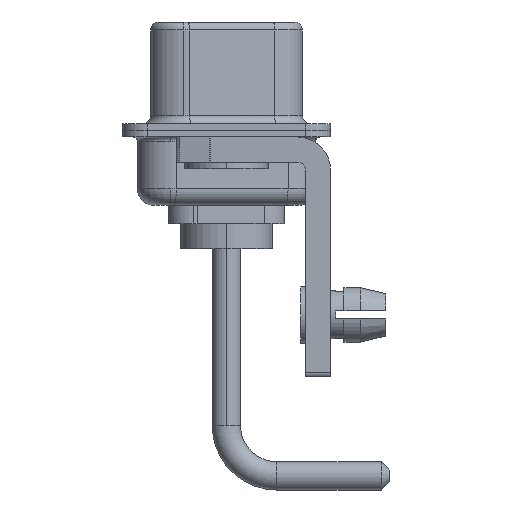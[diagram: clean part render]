
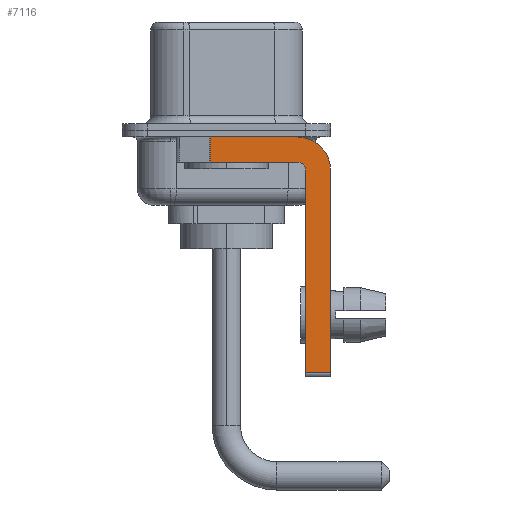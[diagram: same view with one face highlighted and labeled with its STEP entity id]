
A CAD part, left-side view. The second image highlights one B-rep face of the part: STEP entity #7116.
In plain terms, the highlighted planar face has unit normal (-1, 0, 0).
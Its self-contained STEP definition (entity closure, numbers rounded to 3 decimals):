
#137 = CARTESIAN_POINT ( 'NONE',  ( -2.9, -4.75, -14.55 ) ) ;
#662 = AXIS2_PLACEMENT_3D ( 'NONE', #3367, #9069, #10191 ) ;
#943 = CIRCLE ( 'NONE', #3325, 0.5 ) ;
#1096 = CARTESIAN_POINT ( 'NONE',  ( -2.9, -6.25, -2.4 ) ) ;
#1313 = CARTESIAN_POINT ( 'NONE',  ( -2.9, -4.75, -2.4 ) ) ;
#1391 = DIRECTION ( 'NONE',  ( 0., -1., 0. ) ) ;
#1583 = VERTEX_POINT ( 'NONE', #15794 ) ;
#1689 = EDGE_CURVE ( 'NONE', #6474, #12351, #4305, .T. ) ;
#1691 = VERTEX_POINT ( 'NONE', #13336 ) ;
#1703 = CARTESIAN_POINT ( 'NONE',  ( -2.9, -4.25, -2.4 ) ) ;
#1870 = FACE_OUTER_BOUND ( 'NONE', #11598, .T. ) ;
#2334 = EDGE_CURVE ( 'NONE', #17077, #16616, #3514, .T. ) ;
#2384 = ORIENTED_EDGE ( 'NONE', *, *, #13495, .F. ) ;
#2458 = LINE ( 'NONE', #12449, #12883 ) ;
#3183 = DIRECTION ( 'NONE',  ( 1., 0., 0. ) ) ;
#3325 = AXIS2_PLACEMENT_3D ( 'NONE', #5732, #7036, #17232 ) ;
#3367 = CARTESIAN_POINT ( 'NONE',  ( -2.9, -4.25, -2.4 ) ) ;
#3404 = ORIENTED_EDGE ( 'NONE', *, *, #1689, .F. ) ;
#3514 = LINE ( 'NONE', #1096, #5701 ) ;
#3621 = LINE ( 'NONE', #9499, #6588 ) ;
#4081 = DIRECTION ( 'NONE',  ( 0., -1., 0. ) ) ;
#4305 = LINE ( 'NONE', #8596, #7178 ) ;
#4369 = CARTESIAN_POINT ( 'NONE',  ( -2.9, 3., -0.4 ) ) ;
#5701 = VECTOR ( 'NONE', #16592, 1000. ) ;
#5732 = CARTESIAN_POINT ( 'NONE',  ( -2.9, -4.25, -2.4 ) ) ;
#5976 = CARTESIAN_POINT ( 'NONE',  ( -2.9, -6.25, -14.55 ) ) ;
#6071 = ORIENTED_EDGE ( 'NONE', *, *, #2334, .F. ) ;
#6303 = VECTOR ( 'NONE', #1391, 1000. ) ;
#6474 = VERTEX_POINT ( 'NONE', #137 ) ;
#6588 = VECTOR ( 'NONE', #4081, 1000. ) ;
#7036 = DIRECTION ( 'NONE',  ( -1., 0., 0. ) ) ;
#7116 = ADVANCED_FACE ( 'NONE', ( #1870 ), #16073, .F. ) ;
#7178 = VECTOR ( 'NONE', #14293, 1000. ) ;
#7444 = CARTESIAN_POINT ( 'NONE',  ( -2.9, -6.25, -2.4 ) ) ;
#7751 = CARTESIAN_POINT ( 'NONE',  ( -2.9, -4.25, -0.4 ) ) ;
#8210 = EDGE_CURVE ( 'NONE', #1691, #1583, #9915, .T. ) ;
#8596 = CARTESIAN_POINT ( 'NONE',  ( -2.9, -4.75, -14.8 ) ) ;
#9069 = DIRECTION ( 'NONE',  ( 1., 0., 0. ) ) ;
#9499 = CARTESIAN_POINT ( 'NONE',  ( -2.9, -4.25, -14.55 ) ) ;
#9915 = LINE ( 'NONE', #11332, #17137 ) ;
#9967 = LINE ( 'NONE', #4369, #6303 ) ;
#10090 = AXIS2_PLACEMENT_3D ( 'NONE', #1703, #3183, #16254 ) ;
#10164 = EDGE_CURVE ( 'NONE', #6474, #16616, #3621, .T. ) ;
#10191 = DIRECTION ( 'NONE',  ( 0., 0., -1. ) ) ;
#11332 = CARTESIAN_POINT ( 'NONE',  ( -2.9, 0.978, -1.9 ) ) ;
#11598 = EDGE_LOOP ( 'NONE', ( #2384, #15043, #16427, #17782, #3404, #17069, #6071, #17794 ) ) ;
#12181 = VERTEX_POINT ( 'NONE', #7751 ) ;
#12351 = VERTEX_POINT ( 'NONE', #1313 ) ;
#12449 = CARTESIAN_POINT ( 'NONE',  ( -2.9, -4.25, -1.9 ) ) ;
#12548 = DIRECTION ( 'NONE',  ( 0., 0., -1. ) ) ;
#12632 = CARTESIAN_POINT ( 'NONE',  ( -2.9, -4.25, -1.9 ) ) ;
#12883 = VECTOR ( 'NONE', #13757, 1000. ) ;
#13336 = CARTESIAN_POINT ( 'NONE',  ( -2.9, 0.978, -0.4 ) ) ;
#13495 = EDGE_CURVE ( 'NONE', #1691, #12181, #9967, .T. ) ;
#13757 = DIRECTION ( 'NONE',  ( 0., 1., 0. ) ) ;
#14137 = EDGE_CURVE ( 'NONE', #14305, #1583, #2458, .T. ) ;
#14245 = EDGE_CURVE ( 'NONE', #12351, #14305, #943, .T. ) ;
#14293 = DIRECTION ( 'NONE',  ( 0., 0., 1. ) ) ;
#14305 = VERTEX_POINT ( 'NONE', #12632 ) ;
#14500 = EDGE_CURVE ( 'NONE', #12181, #17077, #16785, .T. ) ;
#15043 = ORIENTED_EDGE ( 'NONE', *, *, #8210, .T. ) ;
#15794 = CARTESIAN_POINT ( 'NONE',  ( -2.9, 0.978, -1.9 ) ) ;
#16073 = PLANE ( 'NONE',  #10090 ) ;
#16254 = DIRECTION ( 'NONE',  ( 0., 0., -1. ) ) ;
#16427 = ORIENTED_EDGE ( 'NONE', *, *, #14137, .F. ) ;
#16592 = DIRECTION ( 'NONE',  ( 0., 0., -1. ) ) ;
#16616 = VERTEX_POINT ( 'NONE', #5976 ) ;
#16785 = CIRCLE ( 'NONE', #662, 2. ) ;
#17069 = ORIENTED_EDGE ( 'NONE', *, *, #10164, .T. ) ;
#17077 = VERTEX_POINT ( 'NONE', #7444 ) ;
#17137 = VECTOR ( 'NONE', #12548, 1000. ) ;
#17232 = DIRECTION ( 'NONE',  ( 0., 0., 1. ) ) ;
#17782 = ORIENTED_EDGE ( 'NONE', *, *, #14245, .F. ) ;
#17794 = ORIENTED_EDGE ( 'NONE', *, *, #14500, .F. ) ;
